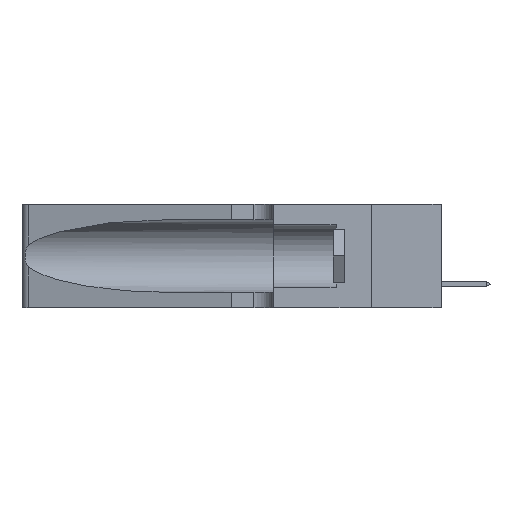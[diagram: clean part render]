
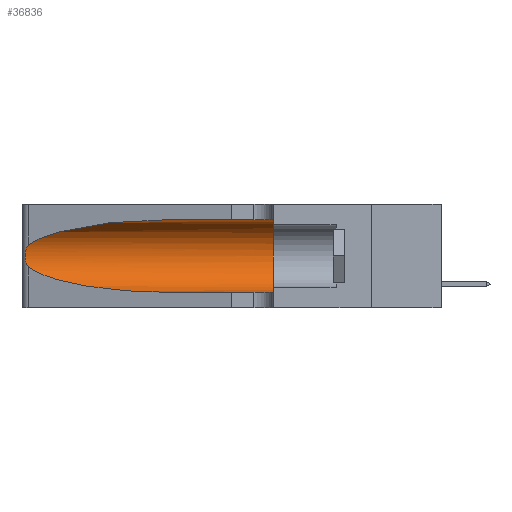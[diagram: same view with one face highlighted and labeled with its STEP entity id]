
A CAD part, left-side view. The second image highlights one B-rep face of the part: STEP entity #36836.
In plain terms, the highlighted cylindrical face has radius 3.308 mm (diameter 6.617 mm), a partial arc.
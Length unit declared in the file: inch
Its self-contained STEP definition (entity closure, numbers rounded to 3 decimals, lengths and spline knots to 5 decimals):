
#111 = VERTEX_POINT ( 'NONE', #15144 ) ;
#341 = CARTESIAN_POINT ( 'NONE',  ( 0.26018, 1.23835, 0.19895 ) ) ;
#384 = EDGE_CURVE ( 'NONE', #37048, #111, #8305, .T. ) ;
#477 =( BOUNDED_CURVE ( )  B_SPLINE_CURVE ( 3, ( #23429, #17268, #10448, #40654 ),
 .UNSPECIFIED., .F., .F. ) 
 B_SPLINE_CURVE_WITH_KNOTS ( ( 4, 4 ),
 ( 3.44316, 4.71239 ),
 .UNSPECIFIED. ) 
 CURVE ( )  GEOMETRIC_REPRESENTATION_ITEM ( )  RATIONAL_B_SPLINE_CURVE ( ( 1., 0.87, 0.87, 1. ) ) 
 REPRESENTATION_ITEM ( '' )  );
#480 = CARTESIAN_POINT ( 'NONE',  ( 0.25856, 1.23593, 0.16098 ) ) ;
#726 = ORIENTED_EDGE ( 'NONE', *, *, #384, .T. ) ;
#857 = CARTESIAN_POINT ( 'NONE',  ( 0.1305, 0.35, 0.05475 ) ) ;
#1223 = CARTESIAN_POINT ( 'NONE',  ( 0.25487, 1.22718, 0.14631 ) ) ;
#1245 = CARTESIAN_POINT ( 'NONE',  ( 0.1305, 0.35, 0.185 ) ) ;
#1385 = DIRECTION ( 'NONE',  ( 0., 1., 0. ) ) ;
#1990 = AXIS2_PLACEMENT_3D ( 'NONE', #1245, #1385, #11468 ) ;
#2422 = AXIS2_PLACEMENT_3D ( 'NONE', #29615, #39625, #13156 ) ;
#3365 = VERTEX_POINT ( 'NONE', #28909 ) ;
#3574 = CARTESIAN_POINT ( 'NONE',  ( 0.25555, 1.22994, 0.2215 ) ) ;
#4251 = EDGE_CURVE ( 'NONE', #26557, #3365, #14170, .T. ) ;
#4782 = EDGE_CURVE ( 'NONE', #111, #19147, #477, .T. ) ;
#4812 = CYLINDRICAL_SURFACE ( 'NONE', #2422, 0.13025 ) ;
#4966 = DIRECTION ( 'NONE',  ( 0., -1., 0. ) ) ;
#7089 = CARTESIAN_POINT ( 'NONE',  ( 0.26075, 1.23896, 0.19203 ) ) ;
#8305 = B_SPLINE_CURVE_WITH_KNOTS ( 'NONE', 3,
 ( #36891, #3574, #37014, #16978, #20344, #341, #7089, #30376, #17112, #480, #27731, #27592, #33956, #1223 ),
 .UNSPECIFIED., .F., .F.,
 ( 4, 2, 2, 2, 2, 2, 4 ),
 ( 0., 0.00027, 0.00053, 0.00107, 0.0016, 0.00187, 0.00214 ),
 .UNSPECIFIED. ) ;
#9707 = ORIENTED_EDGE ( 'NONE', *, *, #4251, .F. ) ;
#10122 = EDGE_CURVE ( 'NONE', #19147, #10645, #16617, .T. ) ;
#10448 = CARTESIAN_POINT ( 'NONE',  ( 0.18966, 0.96281, 0.05475 ) ) ;
#10523 = FACE_OUTER_BOUND ( 'NONE', #42978, .T. ) ;
#10645 = VERTEX_POINT ( 'NONE', #857 ) ;
#10844 = VECTOR ( 'NONE', #22119, 39.37008 ) ;
#11319 = ORIENTED_EDGE ( 'NONE', *, *, #4782, .T. ) ;
#11468 = DIRECTION ( 'NONE',  ( 0., 0., 1. ) ) ;
#13156 = DIRECTION ( 'NONE',  ( 0., 0., -1. ) ) ;
#14170 = LINE ( 'NONE', #39921, #41231 ) ;
#15144 = CARTESIAN_POINT ( 'NONE',  ( 0.25487, 1.22718, 0.14631 ) ) ;
#15402 = CARTESIAN_POINT ( 'NONE',  ( 0.1305, 1.61858, 0.05475 ) ) ;
#16349 = EDGE_CURVE ( 'NONE', #3365, #10645, #20148, .T. ) ;
#16617 = LINE ( 'NONE', #15402, #10844 ) ;
#16978 = CARTESIAN_POINT ( 'NONE',  ( 0.25787, 1.23484, 0.2124 ) ) ;
#17112 = CARTESIAN_POINT ( 'NONE',  ( 0.26017, 1.23833, 0.17102 ) ) ;
#17268 = CARTESIAN_POINT ( 'NONE',  ( 0.2373, 1.15595, 0.08982 ) ) ;
#17441 = ORIENTED_EDGE ( 'NONE', *, *, #10122, .T. ) ;
#18748 = CARTESIAN_POINT ( 'NONE',  ( 0.25487, 1.22718, 0.22369 ) ) ;
#19147 = VERTEX_POINT ( 'NONE', #24786 ) ;
#20148 = CIRCLE ( 'NONE', #1990, 0.13025 ) ;
#20344 = CARTESIAN_POINT ( 'NONE',  ( 0.25854, 1.2359, 0.20912 ) ) ;
#22119 = DIRECTION ( 'NONE',  ( 0., -1., 0. ) ) ;
#23429 = CARTESIAN_POINT ( 'NONE',  ( 0.25487, 1.22718, 0.14631 ) ) ;
#24786 = CARTESIAN_POINT ( 'NONE',  ( 0.1305, 0.72297, 0.05475 ) ) ;
#26557 = VERTEX_POINT ( 'NONE', #31252 ) ;
#27195 =( BOUNDED_CURVE ( )  B_SPLINE_CURVE ( 3, ( #29072, #29215, #35766, #18748 ),
 .UNSPECIFIED., .F., .F. ) 
 B_SPLINE_CURVE_WITH_KNOTS ( ( 4, 4 ),
 ( 1.5708, 2.84003 ),
 .UNSPECIFIED. ) 
 CURVE ( )  GEOMETRIC_REPRESENTATION_ITEM ( )  RATIONAL_B_SPLINE_CURVE ( ( 1., 0.87, 0.87, 1. ) ) 
 REPRESENTATION_ITEM ( '' )  );
#27592 = CARTESIAN_POINT ( 'NONE',  ( 0.25639, 1.23186, 0.15144 ) ) ;
#27731 = CARTESIAN_POINT ( 'NONE',  ( 0.25789, 1.23486, 0.15765 ) ) ;
#28909 = CARTESIAN_POINT ( 'NONE',  ( 0.1305, 0.35, 0.31525 ) ) ;
#29072 = CARTESIAN_POINT ( 'NONE',  ( 0.1305, 0.72297, 0.31525 ) ) ;
#29215 = CARTESIAN_POINT ( 'NONE',  ( 0.18966, 0.96281, 0.31525 ) ) ;
#29615 = CARTESIAN_POINT ( 'NONE',  ( 0.1305, 1.61858, 0.185 ) ) ;
#30376 = CARTESIAN_POINT ( 'NONE',  ( 0.26075, 1.23896, 0.178 ) ) ;
#31252 = CARTESIAN_POINT ( 'NONE',  ( 0.1305, 0.72297, 0.31525 ) ) ;
#33956 = CARTESIAN_POINT ( 'NONE',  ( 0.25555, 1.22993, 0.14849 ) ) ;
#35242 = ORIENTED_EDGE ( 'NONE', *, *, #16349, .F. ) ;
#35402 = EDGE_CURVE ( 'NONE', #26557, #37048, #27195, .T. ) ;
#35766 = CARTESIAN_POINT ( 'NONE',  ( 0.2373, 1.15595, 0.28018 ) ) ;
#36836 = ADVANCED_FACE ( 'NONE', ( #10523 ), #4812, .F. ) ;
#36891 = CARTESIAN_POINT ( 'NONE',  ( 0.25487, 1.22718, 0.22369 ) ) ;
#37014 = CARTESIAN_POINT ( 'NONE',  ( 0.25639, 1.23184, 0.21858 ) ) ;
#37048 = VERTEX_POINT ( 'NONE', #37585 ) ;
#37585 = CARTESIAN_POINT ( 'NONE',  ( 0.25487, 1.22718, 0.22369 ) ) ;
#39625 = DIRECTION ( 'NONE',  ( 0., -1., 0. ) ) ;
#39921 = CARTESIAN_POINT ( 'NONE',  ( 0.1305, 1.61858, 0.31525 ) ) ;
#40654 = CARTESIAN_POINT ( 'NONE',  ( 0.1305, 0.72297, 0.05475 ) ) ;
#41231 = VECTOR ( 'NONE', #4966, 39.37008 ) ;
#41527 = ORIENTED_EDGE ( 'NONE', *, *, #35402, .T. ) ;
#42978 = EDGE_LOOP ( 'NONE', ( #41527, #726, #11319, #17441, #35242, #9707 ) ) ;
